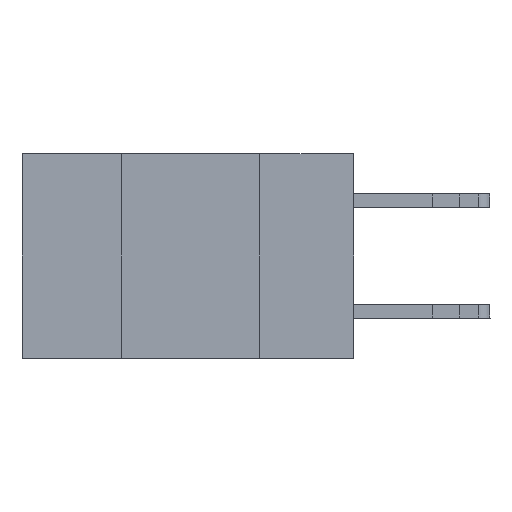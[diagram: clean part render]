
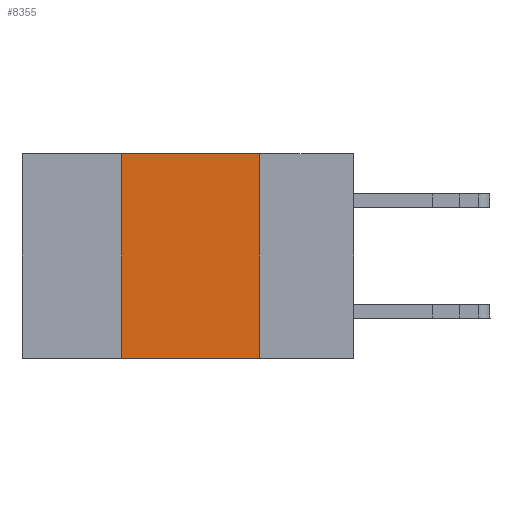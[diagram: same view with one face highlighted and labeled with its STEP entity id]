
A CAD part, left-side view. The second image highlights one B-rep face of the part: STEP entity #8355.
In plain terms, the highlighted planar face has unit normal (-1, 0, 0).
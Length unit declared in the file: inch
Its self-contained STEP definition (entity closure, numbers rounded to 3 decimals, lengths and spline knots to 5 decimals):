
#342 = ORIENTED_EDGE ( 'NONE', *, *, #20500, .T. ) ;
#830 = CARTESIAN_POINT ( 'NONE',  ( 0., 0.17, 0. ) ) ;
#1969 = VECTOR ( 'NONE', #6049, 39.37008 ) ;
#4404 = ORIENTED_EDGE ( 'NONE', *, *, #33578, .F. ) ;
#5283 = DIRECTION ( 'NONE',  ( 1., 0., 0. ) ) ;
#5602 = VECTOR ( 'NONE', #33194, 39.37008 ) ;
#6049 = DIRECTION ( 'NONE',  ( 0., 0., -1. ) ) ;
#7919 = EDGE_LOOP ( 'NONE', ( #27263, #4404, #29188, #342 ) ) ;
#8355 = ADVANCED_FACE ( 'NONE', ( #22007 ), #24803, .F. ) ;
#8879 = LINE ( 'NONE', #11849, #14797 ) ;
#11114 = EDGE_CURVE ( 'NONE', #26231, #17297, #20942, .T. ) ;
#11849 = CARTESIAN_POINT ( 'NONE',  ( 0., 0.6, 0. ) ) ;
#13353 = DIRECTION ( 'NONE',  ( 0., 0., -1. ) ) ;
#14797 = VECTOR ( 'NONE', #16452, 39.37008 ) ;
#16452 = DIRECTION ( 'NONE',  ( 0., -1., 0. ) ) ;
#16962 = CARTESIAN_POINT ( 'NONE',  ( 0., 0.17, 0. ) ) ;
#17297 = VERTEX_POINT ( 'NONE', #27791 ) ;
#19925 = CARTESIAN_POINT ( 'NONE',  ( 0., 0.42, -0.37 ) ) ;
#19965 = LINE ( 'NONE', #16962, #1969 ) ;
#20014 = DIRECTION ( 'NONE',  ( 0., -1., 0. ) ) ;
#20500 = EDGE_CURVE ( 'NONE', #26231, #23909, #20546, .T. ) ;
#20546 = LINE ( 'NONE', #27753, #30460 ) ;
#20942 = LINE ( 'NONE', #31652, #5602 ) ;
#22007 = FACE_OUTER_BOUND ( 'NONE', #7919, .T. ) ;
#23637 = AXIS2_PLACEMENT_3D ( 'NONE', #32360, #5283, #13353 ) ;
#23909 = VERTEX_POINT ( 'NONE', #25740 ) ;
#24803 = PLANE ( 'NONE',  #23637 ) ;
#25588 = EDGE_CURVE ( 'NONE', #29991, #23909, #19965, .T. ) ;
#25740 = CARTESIAN_POINT ( 'NONE',  ( 0., 0.17, -0.37 ) ) ;
#26231 = VERTEX_POINT ( 'NONE', #19925 ) ;
#27263 = ORIENTED_EDGE ( 'NONE', *, *, #25588, .F. ) ;
#27753 = CARTESIAN_POINT ( 'NONE',  ( 0., 0.6, -0.37 ) ) ;
#27791 = CARTESIAN_POINT ( 'NONE',  ( 0., 0.42, 0. ) ) ;
#29188 = ORIENTED_EDGE ( 'NONE', *, *, #11114, .F. ) ;
#29991 = VERTEX_POINT ( 'NONE', #830 ) ;
#30460 = VECTOR ( 'NONE', #20014, 39.37008 ) ;
#31652 = CARTESIAN_POINT ( 'NONE',  ( 0., 0.42, 0. ) ) ;
#32360 = CARTESIAN_POINT ( 'NONE',  ( 0., 0.6, 0. ) ) ;
#33194 = DIRECTION ( 'NONE',  ( 0., 0., 1. ) ) ;
#33578 = EDGE_CURVE ( 'NONE', #17297, #29991, #8879, .T. ) ;
